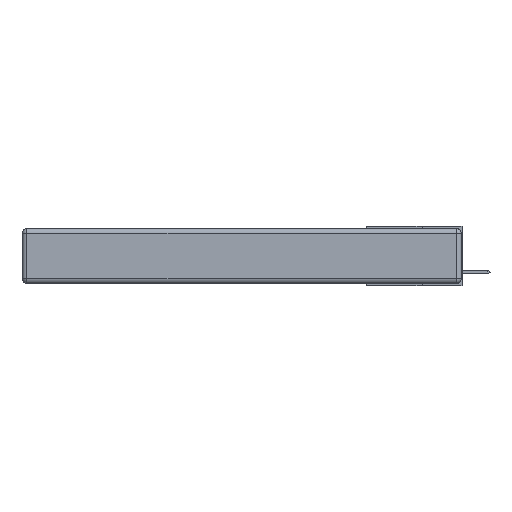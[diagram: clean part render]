
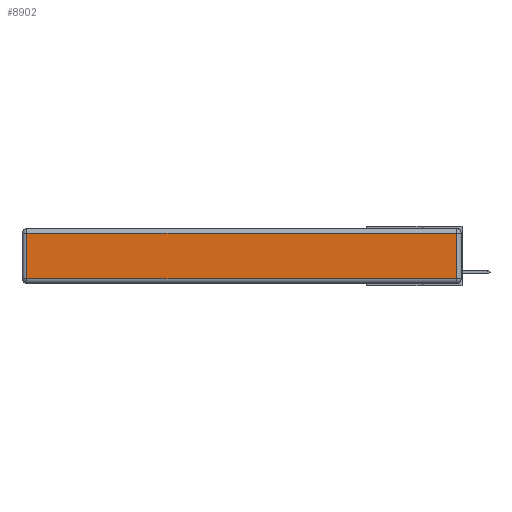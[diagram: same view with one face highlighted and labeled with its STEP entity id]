
A CAD part, left-side view. The second image highlights one B-rep face of the part: STEP entity #8902.
In plain terms, the highlighted planar face has unit normal (-1, 0, 0).
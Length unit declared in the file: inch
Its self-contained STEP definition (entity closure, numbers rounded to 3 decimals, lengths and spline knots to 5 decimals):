
#503 = LINE ( 'NONE', #5709, #12310 ) ;
#1264 = ORIENTED_EDGE ( 'NONE', *, *, #15211, .T. ) ;
#3353 = ORIENTED_EDGE ( 'NONE', *, *, #16336, .T. ) ;
#3973 = DIRECTION ( 'NONE',  ( 0., -1., 0. ) ) ;
#3991 = ORIENTED_EDGE ( 'NONE', *, *, #16414, .T. ) ;
#4360 = ORIENTED_EDGE ( 'NONE', *, *, #6032, .T. ) ;
#4563 = LINE ( 'NONE', #9008, #8794 ) ;
#5063 = DIRECTION ( 'NONE',  ( 0., 1., 0. ) ) ;
#5117 = CARTESIAN_POINT ( 'NONE',  ( 0., 0., -0.313 ) ) ;
#5709 = CARTESIAN_POINT ( 'NONE',  ( 0., 2.72, -0.343 ) ) ;
#6032 = EDGE_CURVE ( 'NONE', #15495, #9713, #4563, .T. ) ;
#6561 = DIRECTION ( 'NONE',  ( 0., 0., 1. ) ) ;
#7797 = FACE_OUTER_BOUND ( 'NONE', #17445, .T. ) ;
#8217 = DIRECTION ( 'NONE',  ( 0., 0., -1. ) ) ;
#8567 = VERTEX_POINT ( 'NONE', #15088 ) ;
#8794 = VECTOR ( 'NONE', #5063, 39.37008 ) ;
#8843 = DIRECTION ( 'NONE',  ( -1., 0., 0. ) ) ;
#8902 = ADVANCED_FACE ( 'NONE', ( #7797 ), #11298, .T. ) ;
#9008 = CARTESIAN_POINT ( 'NONE',  ( 0., 2.75, -0.03 ) ) ;
#9154 = VECTOR ( 'NONE', #6561, 39.37008 ) ;
#9327 = AXIS2_PLACEMENT_3D ( 'NONE', #11417, #8843, #10169 ) ;
#9713 = VERTEX_POINT ( 'NONE', #15470 ) ;
#10169 = DIRECTION ( 'NONE',  ( 0., 0., 1. ) ) ;
#11298 = PLANE ( 'NONE',  #9327 ) ;
#11417 = CARTESIAN_POINT ( 'NONE',  ( 0., 0., -0.343 ) ) ;
#12095 = LINE ( 'NONE', #5117, #16106 ) ;
#12310 = VECTOR ( 'NONE', #8217, 39.37008 ) ;
#12773 = LINE ( 'NONE', #14605, #9154 ) ;
#14605 = CARTESIAN_POINT ( 'NONE',  ( 0., 0.03, -0.343 ) ) ;
#14649 = CARTESIAN_POINT ( 'NONE',  ( 0., 0.03, -0.03 ) ) ;
#15088 = CARTESIAN_POINT ( 'NONE',  ( 0., 0.03, -0.313 ) ) ;
#15152 = CARTESIAN_POINT ( 'NONE',  ( 0., 2.72, -0.313 ) ) ;
#15211 = EDGE_CURVE ( 'NONE', #8567, #15495, #12773, .T. ) ;
#15470 = CARTESIAN_POINT ( 'NONE',  ( 0., 2.72, -0.03 ) ) ;
#15495 = VERTEX_POINT ( 'NONE', #14649 ) ;
#16106 = VECTOR ( 'NONE', #3973, 39.37008 ) ;
#16336 = EDGE_CURVE ( 'NONE', #9713, #17085, #503, .T. ) ;
#16414 = EDGE_CURVE ( 'NONE', #17085, #8567, #12095, .T. ) ;
#17085 = VERTEX_POINT ( 'NONE', #15152 ) ;
#17445 = EDGE_LOOP ( 'NONE', ( #3991, #1264, #4360, #3353 ) ) ;
